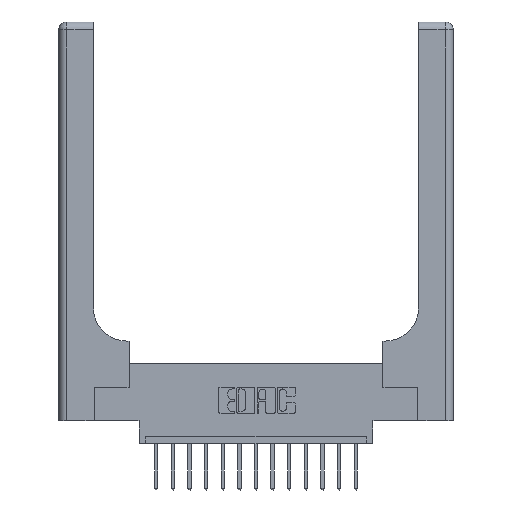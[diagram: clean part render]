
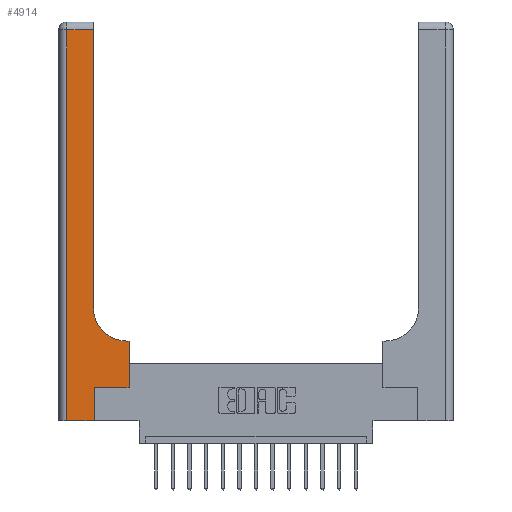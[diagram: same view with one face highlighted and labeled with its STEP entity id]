
A CAD part, top view. The second image highlights one B-rep face of the part: STEP entity #4914.
In plain terms, the highlighted planar face has unit normal (0, 0, 1).
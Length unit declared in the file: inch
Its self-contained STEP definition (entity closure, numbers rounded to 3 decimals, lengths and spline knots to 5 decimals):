
#57 = ORIENTED_EDGE ( 'NONE', *, *, #16482, .T. ) ;
#354 = FACE_OUTER_BOUND ( 'NONE', #12405, .T. ) ;
#734 = ORIENTED_EDGE ( 'NONE', *, *, #14167, .T. ) ;
#965 = DIRECTION ( 'NONE',  ( 0., 1., 0. ) ) ;
#1096 = CARTESIAN_POINT ( 'NONE',  ( 0.06, 2.94, 0.37 ) ) ;
#1555 = VERTEX_POINT ( 'NONE', #9978 ) ;
#2185 = DIRECTION ( 'NONE',  ( 0., 0., -1. ) ) ;
#2204 = ORIENTED_EDGE ( 'NONE', *, *, #2893, .T. ) ;
#2351 = DIRECTION ( 'NONE',  ( 1., 0., 0. ) ) ;
#2483 = VECTOR ( 'NONE', #12138, 39.37008 ) ;
#2684 = VERTEX_POINT ( 'NONE', #14392 ) ;
#2893 = EDGE_CURVE ( 'NONE', #10501, #1555, #10758, .T. ) ;
#3161 = LINE ( 'NONE', #12909, #13186 ) ;
#3238 = VECTOR ( 'NONE', #10937, 39.37008 ) ;
#3342 = EDGE_CURVE ( 'NONE', #15044, #8244, #11488, .T. ) ;
#3612 = AXIS2_PLACEMENT_3D ( 'NONE', #16385, #11267, #16558 ) ;
#3656 = VECTOR ( 'NONE', #13200, 39.37008 ) ;
#3681 = VECTOR ( 'NONE', #14209, 39.37008 ) ;
#4037 = VERTEX_POINT ( 'NONE', #9160 ) ;
#4669 = ORIENTED_EDGE ( 'NONE', *, *, #17060, .T. ) ;
#4679 = LINE ( 'NONE', #5592, #3238 ) ;
#4738 = CARTESIAN_POINT ( 'NONE',  ( 0.51, 0.85, 0.37 ) ) ;
#4818 = ORIENTED_EDGE ( 'NONE', *, *, #3342, .T. ) ;
#4914 = ADVANCED_FACE ( 'NONE', ( #354 ), #15278, .F. ) ;
#5592 = CARTESIAN_POINT ( 'NONE',  ( 0.528, 0.25, 0.37 ) ) ;
#5846 = VERTEX_POINT ( 'NONE', #7203 ) ;
#6045 = DIRECTION ( 'NONE',  ( 0., -1., 0. ) ) ;
#6167 = LINE ( 'NONE', #8816, #3681 ) ;
#7203 = CARTESIAN_POINT ( 'NONE',  ( 0.26, 0.85, 0.37 ) ) ;
#8244 = VERTEX_POINT ( 'NONE', #1096 ) ;
#8448 = VECTOR ( 'NONE', #965, 39.37008 ) ;
#8622 = CARTESIAN_POINT ( 'NONE',  ( 0.265, 0., 0.37 ) ) ;
#8738 = CIRCLE ( 'NONE', #11209, 0.25 ) ;
#8816 = CARTESIAN_POINT ( 'NONE',  ( 0.265, 0., 0.37 ) ) ;
#8915 = VERTEX_POINT ( 'NONE', #9539 ) ;
#8959 = EDGE_CURVE ( 'NONE', #14877, #4037, #6167, .T. ) ;
#9058 = EDGE_CURVE ( 'NONE', #5846, #15044, #12449, .T. ) ;
#9067 = LINE ( 'NONE', #15755, #3656 ) ;
#9085 = CARTESIAN_POINT ( 'NONE',  ( 0.528, 0.6, 0.37 ) ) ;
#9160 = CARTESIAN_POINT ( 'NONE',  ( 0.265, 0.25, 0.37 ) ) ;
#9539 = CARTESIAN_POINT ( 'NONE',  ( 0.528, 0.25, 0.37 ) ) ;
#9978 = CARTESIAN_POINT ( 'NONE',  ( 0.51, 0.6, 0.37 ) ) ;
#10501 = VERTEX_POINT ( 'NONE', #9085 ) ;
#10758 = LINE ( 'NONE', #14918, #13253 ) ;
#10785 = CARTESIAN_POINT ( 'NONE',  ( 0., 2.94, 0.37 ) ) ;
#10937 = DIRECTION ( 'NONE',  ( 0., 1., 0. ) ) ;
#11209 = AXIS2_PLACEMENT_3D ( 'NONE', #4738, #2185, #15377 ) ;
#11267 = DIRECTION ( 'NONE',  ( 0., 0., -1. ) ) ;
#11488 = LINE ( 'NONE', #10785, #2483 ) ;
#11697 = EDGE_CURVE ( 'NONE', #4037, #8915, #3161, .T. ) ;
#12138 = DIRECTION ( 'NONE',  ( -1., 0., 0. ) ) ;
#12405 = EDGE_LOOP ( 'NONE', ( #15288, #4818, #57, #734, #13011, #12558, #15484, #2204, #4669 ) ) ;
#12449 = LINE ( 'NONE', #15533, #8448 ) ;
#12558 = ORIENTED_EDGE ( 'NONE', *, *, #11697, .T. ) ;
#12909 = CARTESIAN_POINT ( 'NONE',  ( 0.265, 0.25, 0.37 ) ) ;
#13011 = ORIENTED_EDGE ( 'NONE', *, *, #8959, .T. ) ;
#13186 = VECTOR ( 'NONE', #2351, 39.37008 ) ;
#13200 = DIRECTION ( 'NONE',  ( 1., 0., 0. ) ) ;
#13253 = VECTOR ( 'NONE', #13572, 39.37008 ) ;
#13572 = DIRECTION ( 'NONE',  ( -1., 0., 0. ) ) ;
#13849 = EDGE_CURVE ( 'NONE', #8915, #10501, #4679, .T. ) ;
#14167 = EDGE_CURVE ( 'NONE', #2684, #14877, #9067, .T. ) ;
#14209 = DIRECTION ( 'NONE',  ( 0., 1., 0. ) ) ;
#14392 = CARTESIAN_POINT ( 'NONE',  ( 0.06, 0., 0.37 ) ) ;
#14876 = VECTOR ( 'NONE', #6045, 39.37008 ) ;
#14877 = VERTEX_POINT ( 'NONE', #8622 ) ;
#14918 = CARTESIAN_POINT ( 'NONE',  ( 0.26, 0.6, 0.37 ) ) ;
#15044 = VERTEX_POINT ( 'NONE', #15331 ) ;
#15278 = PLANE ( 'NONE',  #3612 ) ;
#15288 = ORIENTED_EDGE ( 'NONE', *, *, #9058, .T. ) ;
#15331 = CARTESIAN_POINT ( 'NONE',  ( 0.26, 2.94, 0.37 ) ) ;
#15377 = DIRECTION ( 'NONE',  ( 1., 0., 0. ) ) ;
#15484 = ORIENTED_EDGE ( 'NONE', *, *, #13849, .T. ) ;
#15533 = CARTESIAN_POINT ( 'NONE',  ( 0.26, 3., 0.37 ) ) ;
#15755 = CARTESIAN_POINT ( 'NONE',  ( 0., 0., 0.37 ) ) ;
#15875 = LINE ( 'NONE', #16855, #14876 ) ;
#16385 = CARTESIAN_POINT ( 'NONE',  ( 0., 3., 0.37 ) ) ;
#16482 = EDGE_CURVE ( 'NONE', #8244, #2684, #15875, .T. ) ;
#16558 = DIRECTION ( 'NONE',  ( -1., 0., 0. ) ) ;
#16855 = CARTESIAN_POINT ( 'NONE',  ( 0.06, 3., 0.37 ) ) ;
#17060 = EDGE_CURVE ( 'NONE', #1555, #5846, #8738, .T. ) ;
